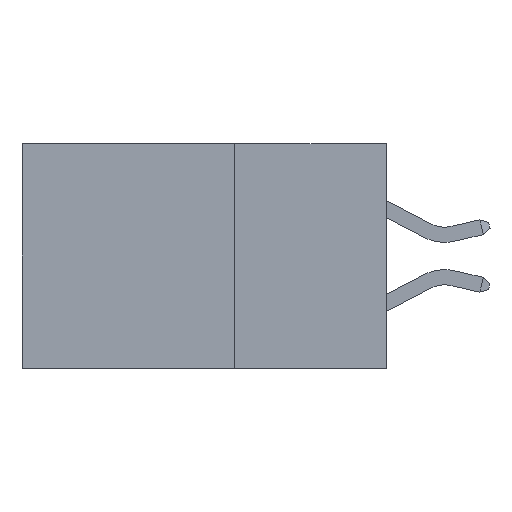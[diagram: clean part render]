
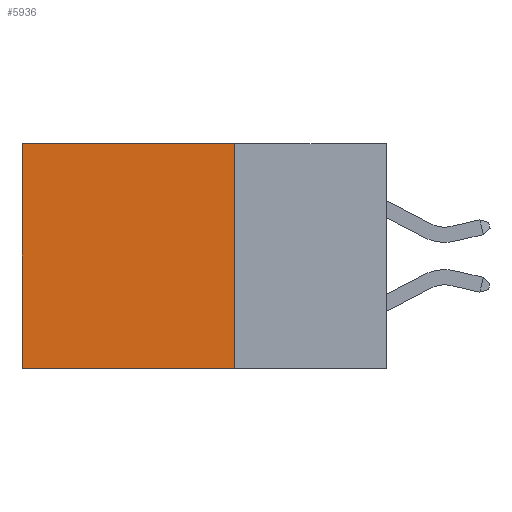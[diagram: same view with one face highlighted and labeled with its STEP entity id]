
A CAD part, left-side view. The second image highlights one B-rep face of the part: STEP entity #5936.
In plain terms, the highlighted planar face has unit normal (-1, 0, 0).
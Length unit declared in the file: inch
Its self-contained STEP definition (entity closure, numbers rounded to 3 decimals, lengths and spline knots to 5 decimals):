
#1920 = LINE ( 'NONE', #12416, #5884 ) ;
#2496 = DIRECTION ( 'NONE',  ( 0., 0., -1. ) ) ;
#3114 = CARTESIAN_POINT ( 'NONE',  ( 0.298, 0.25, 0. ) ) ;
#3955 = VERTEX_POINT ( 'NONE', #4215 ) ;
#4215 = CARTESIAN_POINT ( 'NONE',  ( 0.298, 0.6, 0. ) ) ;
#4371 = VECTOR ( 'NONE', #2496, 39.37008 ) ;
#4678 = DIRECTION ( 'NONE',  ( 0., 1., 0. ) ) ;
#4824 = DIRECTION ( 'NONE',  ( 0., 1., 0. ) ) ;
#4874 = CARTESIAN_POINT ( 'NONE',  ( 0.298, 0.25, 0. ) ) ;
#5449 = AXIS2_PLACEMENT_3D ( 'NONE', #10686, #20355, #10758 ) ;
#5871 = CARTESIAN_POINT ( 'NONE',  ( 0.298, 0.25, 0. ) ) ;
#5883 = PLANE ( 'NONE',  #5449 ) ;
#5884 = VECTOR ( 'NONE', #10844, 39.37008 ) ;
#5936 = ADVANCED_FACE ( 'NONE', ( #18550 ), #5883, .F. ) ;
#7594 = CARTESIAN_POINT ( 'NONE',  ( 0.298, 0.25, -0.37 ) ) ;
#8203 = LINE ( 'NONE', #5871, #4371 ) ;
#8714 = ORIENTED_EDGE ( 'NONE', *, *, #10080, .F. ) ;
#9487 = EDGE_CURVE ( 'NONE', #11924, #3955, #15209, .T. ) ;
#10080 = EDGE_CURVE ( 'NONE', #15036, #14937, #15945, .T. ) ;
#10686 = CARTESIAN_POINT ( 'NONE',  ( 0.298, 0.25, 0. ) ) ;
#10758 = DIRECTION ( 'NONE',  ( 0., 0., -1. ) ) ;
#10844 = DIRECTION ( 'NONE',  ( 0., 0., -1. ) ) ;
#10888 = EDGE_LOOP ( 'NONE', ( #12674, #8714, #16474, #15535 ) ) ;
#11115 = CARTESIAN_POINT ( 'NONE',  ( 0.298, 0.25, -0.37 ) ) ;
#11608 = VECTOR ( 'NONE', #4678, 39.37008 ) ;
#11924 = VERTEX_POINT ( 'NONE', #4874 ) ;
#12416 = CARTESIAN_POINT ( 'NONE',  ( 0.298, 0.6, 0. ) ) ;
#12674 = ORIENTED_EDGE ( 'NONE', *, *, #20344, .T. ) ;
#13194 = EDGE_CURVE ( 'NONE', #11924, #15036, #8203, .T. ) ;
#14706 = VECTOR ( 'NONE', #4824, 39.37008 ) ;
#14937 = VERTEX_POINT ( 'NONE', #17042 ) ;
#15036 = VERTEX_POINT ( 'NONE', #7594 ) ;
#15209 = LINE ( 'NONE', #3114, #14706 ) ;
#15535 = ORIENTED_EDGE ( 'NONE', *, *, #9487, .T. ) ;
#15945 = LINE ( 'NONE', #11115, #11608 ) ;
#16474 = ORIENTED_EDGE ( 'NONE', *, *, #13194, .F. ) ;
#17042 = CARTESIAN_POINT ( 'NONE',  ( 0.298, 0.6, -0.37 ) ) ;
#18550 = FACE_OUTER_BOUND ( 'NONE', #10888, .T. ) ;
#20344 = EDGE_CURVE ( 'NONE', #3955, #14937, #1920, .T. ) ;
#20355 = DIRECTION ( 'NONE',  ( 1., 0., 0. ) ) ;
